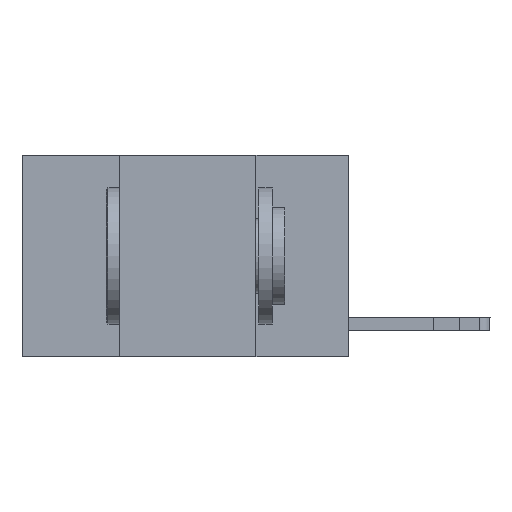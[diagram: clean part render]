
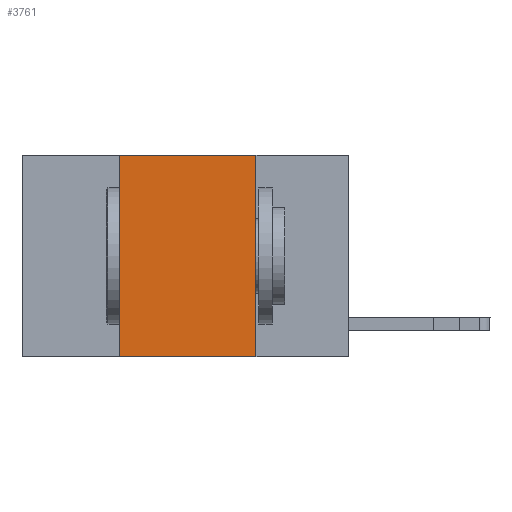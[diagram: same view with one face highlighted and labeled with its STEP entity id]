
A CAD part, left-side view. The second image highlights one B-rep face of the part: STEP entity #3761.
In plain terms, the highlighted planar face has unit normal (-1, 0, 0).
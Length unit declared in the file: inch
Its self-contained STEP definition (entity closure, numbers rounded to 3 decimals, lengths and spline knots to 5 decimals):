
#754 = VECTOR ( 'NONE', #7776, 39.37008 ) ;
#1356 = CARTESIAN_POINT ( 'NONE',  ( 0., 0.6, 0. ) ) ;
#1977 = EDGE_LOOP ( 'NONE', ( #9684, #2590, #9392, #13991 ) ) ;
#2517 = FACE_OUTER_BOUND ( 'NONE', #1977, .T. ) ;
#2590 = ORIENTED_EDGE ( 'NONE', *, *, #14741, .F. ) ;
#3050 = VERTEX_POINT ( 'NONE', #3939 ) ;
#3761 = ADVANCED_FACE ( 'NONE', ( #2517 ), #4871, .F. ) ;
#3939 = CARTESIAN_POINT ( 'NONE',  ( 0., 0.17, 0. ) ) ;
#3942 = CARTESIAN_POINT ( 'NONE',  ( 0., 0.6, -0.37 ) ) ;
#4871 = PLANE ( 'NONE',  #11624 ) ;
#4942 = EDGE_CURVE ( 'NONE', #3050, #8651, #11999, .T. ) ;
#6643 = EDGE_CURVE ( 'NONE', #13251, #9103, #14292, .T. ) ;
#7509 = DIRECTION ( 'NONE',  ( 0., 0., -1. ) ) ;
#7776 = DIRECTION ( 'NONE',  ( 0., -1., 0. ) ) ;
#8329 = DIRECTION ( 'NONE',  ( 1., 0., 0. ) ) ;
#8535 = CARTESIAN_POINT ( 'NONE',  ( 0., 0.42, 0. ) ) ;
#8651 = VERTEX_POINT ( 'NONE', #10203 ) ;
#8766 = DIRECTION ( 'NONE',  ( 0., -1., 0. ) ) ;
#9103 = VERTEX_POINT ( 'NONE', #9882 ) ;
#9392 = ORIENTED_EDGE ( 'NONE', *, *, #6643, .F. ) ;
#9684 = ORIENTED_EDGE ( 'NONE', *, *, #4942, .F. ) ;
#9704 = CARTESIAN_POINT ( 'NONE',  ( 0., 0.17, 0. ) ) ;
#9882 = CARTESIAN_POINT ( 'NONE',  ( 0., 0.42, 0. ) ) ;
#10002 = LINE ( 'NONE', #13616, #754 ) ;
#10203 = CARTESIAN_POINT ( 'NONE',  ( 0., 0.17, -0.37 ) ) ;
#10564 = CARTESIAN_POINT ( 'NONE',  ( 0., 0.42, -0.37 ) ) ;
#10733 = DIRECTION ( 'NONE',  ( 0., 0., 1. ) ) ;
#11020 = LINE ( 'NONE', #3942, #12907 ) ;
#11624 = AXIS2_PLACEMENT_3D ( 'NONE', #1356, #8329, #11757 ) ;
#11757 = DIRECTION ( 'NONE',  ( 0., 0., -1. ) ) ;
#11999 = LINE ( 'NONE', #9704, #14198 ) ;
#12907 = VECTOR ( 'NONE', #8766, 39.37008 ) ;
#12999 = EDGE_CURVE ( 'NONE', #13251, #8651, #11020, .T. ) ;
#13251 = VERTEX_POINT ( 'NONE', #10564 ) ;
#13616 = CARTESIAN_POINT ( 'NONE',  ( 0., 0.6, 0. ) ) ;
#13991 = ORIENTED_EDGE ( 'NONE', *, *, #12999, .T. ) ;
#14040 = VECTOR ( 'NONE', #10733, 39.37008 ) ;
#14198 = VECTOR ( 'NONE', #7509, 39.37008 ) ;
#14292 = LINE ( 'NONE', #8535, #14040 ) ;
#14741 = EDGE_CURVE ( 'NONE', #9103, #3050, #10002, .T. ) ;
